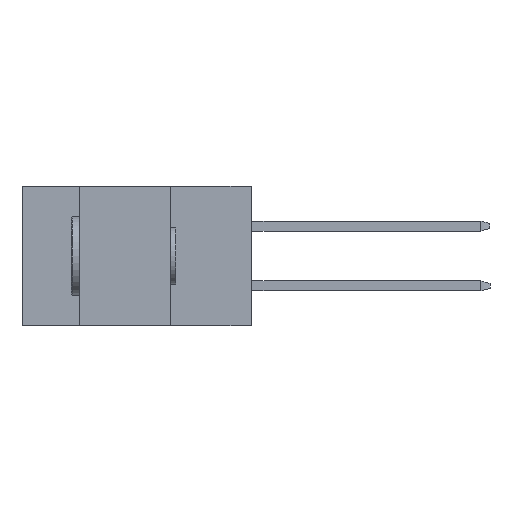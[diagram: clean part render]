
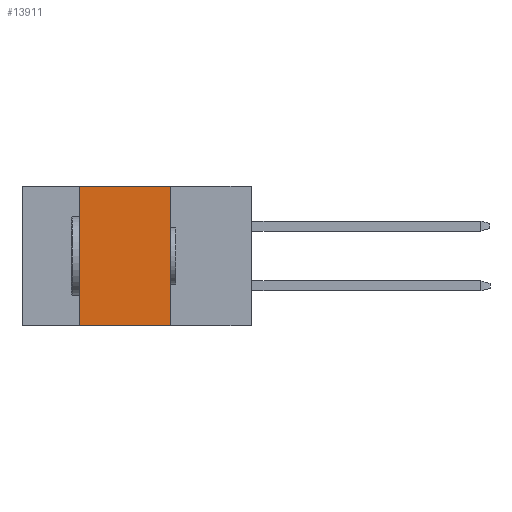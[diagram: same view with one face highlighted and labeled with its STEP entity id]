
A CAD part, left-side view. The second image highlights one B-rep face of the part: STEP entity #13911.
In plain terms, the highlighted planar face has unit normal (-1, 0, 0).
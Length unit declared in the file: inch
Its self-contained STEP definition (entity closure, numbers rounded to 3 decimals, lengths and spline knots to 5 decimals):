
#1226 = PLANE ( 'NONE',  #18929 ) ;
#2214 = ORIENTED_EDGE ( 'NONE', *, *, #2562, .F. ) ;
#2542 = LINE ( 'NONE', #13110, #4941 ) ;
#2562 = EDGE_CURVE ( 'NONE', #9602, #13762, #19447, .T. ) ;
#2630 = EDGE_LOOP ( 'NONE', ( #15997, #17827, #2214, #16707 ) ) ;
#3413 = CARTESIAN_POINT ( 'NONE',  ( 0., 0.254, -0.437 ) ) ;
#3475 = CARTESIAN_POINT ( 'NONE',  ( 0., 0.254, -0.437 ) ) ;
#3762 = LINE ( 'NONE', #9869, #17507 ) ;
#4941 = VECTOR ( 'NONE', #13304, 39.37008 ) ;
#5701 = FACE_OUTER_BOUND ( 'NONE', #2630, .T. ) ;
#5794 = DIRECTION ( 'NONE',  ( 0., 0., -1. ) ) ;
#7275 = CARTESIAN_POINT ( 'NONE',  ( 0., 0.72, 0. ) ) ;
#7333 = DIRECTION ( 'NONE',  ( 0., 0., 1. ) ) ;
#7483 = VERTEX_POINT ( 'NONE', #3413 ) ;
#8372 = VECTOR ( 'NONE', #7333, 39.37008 ) ;
#9498 = LINE ( 'NONE', #3475, #18022 ) ;
#9602 = VERTEX_POINT ( 'NONE', #9865 ) ;
#9865 = CARTESIAN_POINT ( 'NONE',  ( 0., 0.54, -0.437 ) ) ;
#9869 = CARTESIAN_POINT ( 'NONE',  ( 0., 0.72, 0. ) ) ;
#10312 = VERTEX_POINT ( 'NONE', #11087 ) ;
#10787 = EDGE_CURVE ( 'NONE', #13762, #10312, #3762, .T. ) ;
#11087 = CARTESIAN_POINT ( 'NONE',  ( 0., 0.254, 0. ) ) ;
#11190 = EDGE_CURVE ( 'NONE', #9602, #7483, #2542, .T. ) ;
#12261 = CARTESIAN_POINT ( 'NONE',  ( 0., 0.54, -0.437 ) ) ;
#13110 = CARTESIAN_POINT ( 'NONE',  ( 0., 0.72, -0.437 ) ) ;
#13304 = DIRECTION ( 'NONE',  ( 0., -1., 0. ) ) ;
#13762 = VERTEX_POINT ( 'NONE', #14372 ) ;
#13911 = ADVANCED_FACE ( 'NONE', ( #5701 ), #1226, .F. ) ;
#14372 = CARTESIAN_POINT ( 'NONE',  ( 0., 0.54, 0. ) ) ;
#15309 = EDGE_CURVE ( 'NONE', #10312, #7483, #9498, .T. ) ;
#15512 = DIRECTION ( 'NONE',  ( 0., 0., -1. ) ) ;
#15997 = ORIENTED_EDGE ( 'NONE', *, *, #15309, .F. ) ;
#16707 = ORIENTED_EDGE ( 'NONE', *, *, #11190, .T. ) ;
#17507 = VECTOR ( 'NONE', #18935, 39.37008 ) ;
#17827 = ORIENTED_EDGE ( 'NONE', *, *, #10787, .F. ) ;
#18022 = VECTOR ( 'NONE', #15512, 39.37008 ) ;
#18929 = AXIS2_PLACEMENT_3D ( 'NONE', #7275, #19285, #5794 ) ;
#18935 = DIRECTION ( 'NONE',  ( 0., -1., 0. ) ) ;
#19285 = DIRECTION ( 'NONE',  ( 1., 0., 0. ) ) ;
#19447 = LINE ( 'NONE', #12261, #8372 ) ;
